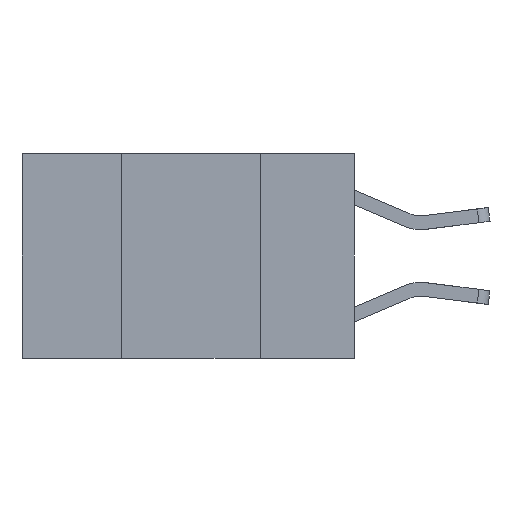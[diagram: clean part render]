
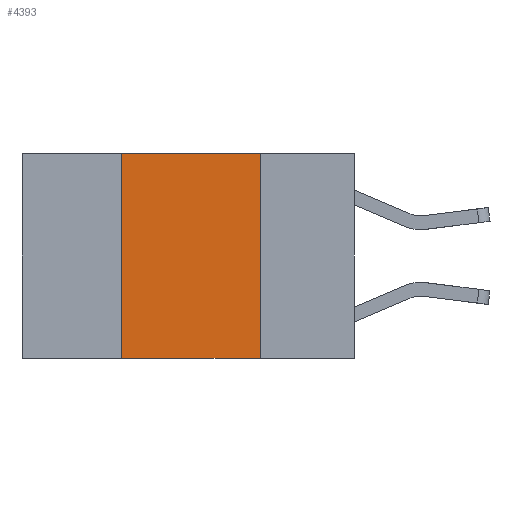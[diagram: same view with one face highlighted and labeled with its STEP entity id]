
A CAD part, left-side view. The second image highlights one B-rep face of the part: STEP entity #4393.
In plain terms, the highlighted planar face has unit normal (-1, 0, 0).
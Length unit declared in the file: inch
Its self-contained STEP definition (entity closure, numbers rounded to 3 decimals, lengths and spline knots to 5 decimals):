
#344 = DIRECTION ( 'NONE',  ( 0., -1., 0. ) ) ;
#453 = EDGE_CURVE ( 'NONE', #2999, #9485, #7745, .T. ) ;
#814 = CARTESIAN_POINT ( 'NONE',  ( 0., 0.42, -0.37 ) ) ;
#1791 = DIRECTION ( 'NONE',  ( 0., 0., 1. ) ) ;
#2287 = CARTESIAN_POINT ( 'NONE',  ( 0., 0.6, 0. ) ) ;
#2507 = EDGE_CURVE ( 'NONE', #5346, #2999, #8695, .T. ) ;
#2643 = VECTOR ( 'NONE', #344, 39.37008 ) ;
#2805 = DIRECTION ( 'NONE',  ( 0., 0., -1. ) ) ;
#2887 = CARTESIAN_POINT ( 'NONE',  ( 0., 0.17, 0. ) ) ;
#2889 = EDGE_LOOP ( 'NONE', ( #3908, #6534, #5633, #7546 ) ) ;
#2999 = VERTEX_POINT ( 'NONE', #4182 ) ;
#3210 = CARTESIAN_POINT ( 'NONE',  ( 0., 0.17, -0.37 ) ) ;
#3339 = CARTESIAN_POINT ( 'NONE',  ( 0., 0.42, 0. ) ) ;
#3727 = VECTOR ( 'NONE', #5376, 39.37008 ) ;
#3761 = VECTOR ( 'NONE', #1791, 39.37008 ) ;
#3908 = ORIENTED_EDGE ( 'NONE', *, *, #7179, .F. ) ;
#4182 = CARTESIAN_POINT ( 'NONE',  ( 0., 0.42, 0. ) ) ;
#4393 = ADVANCED_FACE ( 'NONE', ( #9766 ), #8295, .F. ) ;
#4777 = DIRECTION ( 'NONE',  ( 0., 0., -1. ) ) ;
#4982 = VECTOR ( 'NONE', #4777, 39.37008 ) ;
#5249 = LINE ( 'NONE', #2887, #4982 ) ;
#5346 = VERTEX_POINT ( 'NONE', #814 ) ;
#5376 = DIRECTION ( 'NONE',  ( 0., -1., 0. ) ) ;
#5517 = EDGE_CURVE ( 'NONE', #5346, #8304, #8093, .T. ) ;
#5633 = ORIENTED_EDGE ( 'NONE', *, *, #2507, .F. ) ;
#5784 = CARTESIAN_POINT ( 'NONE',  ( 0., 0.6, -0.37 ) ) ;
#6534 = ORIENTED_EDGE ( 'NONE', *, *, #453, .F. ) ;
#7179 = EDGE_CURVE ( 'NONE', #9485, #8304, #5249, .T. ) ;
#7473 = CARTESIAN_POINT ( 'NONE',  ( 0., 0.6, 0. ) ) ;
#7546 = ORIENTED_EDGE ( 'NONE', *, *, #5517, .T. ) ;
#7745 = LINE ( 'NONE', #2287, #3727 ) ;
#7777 = CARTESIAN_POINT ( 'NONE',  ( 0., 0.17, 0. ) ) ;
#8093 = LINE ( 'NONE', #5784, #2643 ) ;
#8295 = PLANE ( 'NONE',  #9032 ) ;
#8304 = VERTEX_POINT ( 'NONE', #3210 ) ;
#8695 = LINE ( 'NONE', #3339, #3761 ) ;
#9032 = AXIS2_PLACEMENT_3D ( 'NONE', #7473, #9863, #2805 ) ;
#9485 = VERTEX_POINT ( 'NONE', #7777 ) ;
#9766 = FACE_OUTER_BOUND ( 'NONE', #2889, .T. ) ;
#9863 = DIRECTION ( 'NONE',  ( 1., 0., 0. ) ) ;
